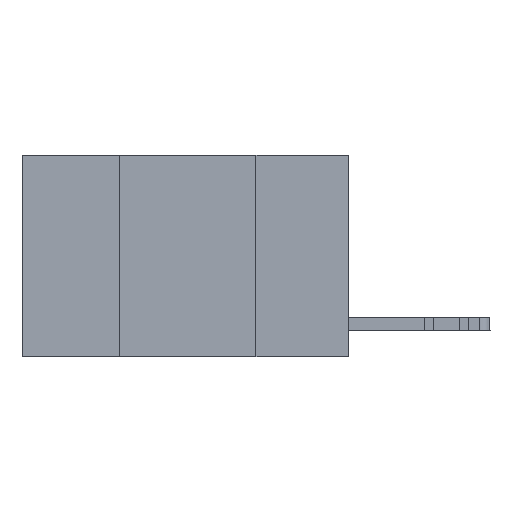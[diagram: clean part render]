
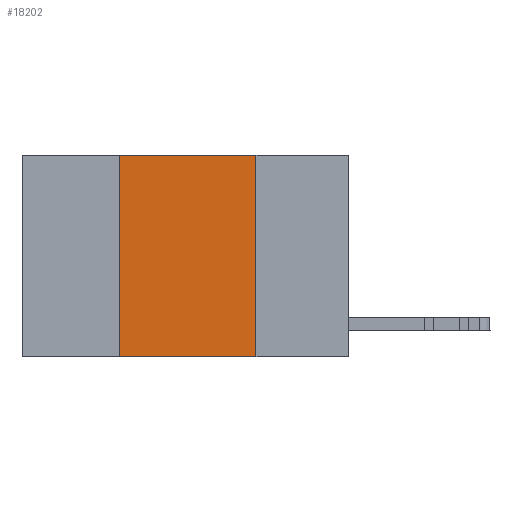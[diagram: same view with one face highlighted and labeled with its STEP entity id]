
A CAD part, left-side view. The second image highlights one B-rep face of the part: STEP entity #18202.
In plain terms, the highlighted planar face has unit normal (-1, 0, 0).
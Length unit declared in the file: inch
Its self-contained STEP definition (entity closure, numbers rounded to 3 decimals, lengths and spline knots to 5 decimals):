
#2142 = LINE ( 'NONE', #16442, #11073 ) ;
#2859 = VERTEX_POINT ( 'NONE', #10514 ) ;
#4257 = ORIENTED_EDGE ( 'NONE', *, *, #20470, .F. ) ;
#4533 = LINE ( 'NONE', #17146, #8910 ) ;
#5981 = PLANE ( 'NONE',  #22032 ) ;
#6725 = LINE ( 'NONE', #23983, #12965 ) ;
#7134 = DIRECTION ( 'NONE',  ( 0., -1., 0. ) ) ;
#8594 = EDGE_LOOP ( 'NONE', ( #9467, #24457, #4257, #24720 ) ) ;
#8910 = VECTOR ( 'NONE', #7134, 39.37008 ) ;
#9030 = CARTESIAN_POINT ( 'NONE',  ( 0., 0.42, -0.37 ) ) ;
#9467 = ORIENTED_EDGE ( 'NONE', *, *, #14985, .F. ) ;
#9581 = LINE ( 'NONE', #13747, #23902 ) ;
#10507 = DIRECTION ( 'NONE',  ( 1., 0., 0. ) ) ;
#10514 = CARTESIAN_POINT ( 'NONE',  ( 0., 0.42, 0. ) ) ;
#11073 = VECTOR ( 'NONE', #25139, 39.37008 ) ;
#11332 = EDGE_CURVE ( 'NONE', #2859, #19741, #4533, .T. ) ;
#12965 = VECTOR ( 'NONE', #14904, 39.37008 ) ;
#13704 = VERTEX_POINT ( 'NONE', #9030 ) ;
#13747 = CARTESIAN_POINT ( 'NONE',  ( 0., 0.6, -0.37 ) ) ;
#14904 = DIRECTION ( 'NONE',  ( 0., 0., -1. ) ) ;
#14985 = EDGE_CURVE ( 'NONE', #19741, #25496, #6725, .T. ) ;
#16442 = CARTESIAN_POINT ( 'NONE',  ( 0., 0.42, 0. ) ) ;
#16849 = CARTESIAN_POINT ( 'NONE',  ( 0., 0.17, -0.37 ) ) ;
#17146 = CARTESIAN_POINT ( 'NONE',  ( 0., 0.6, 0. ) ) ;
#18202 = ADVANCED_FACE ( 'NONE', ( #25062 ), #5981, .F. ) ;
#19572 = CARTESIAN_POINT ( 'NONE',  ( 0., 0.17, 0. ) ) ;
#19741 = VERTEX_POINT ( 'NONE', #19572 ) ;
#20470 = EDGE_CURVE ( 'NONE', #13704, #2859, #2142, .T. ) ;
#20626 = DIRECTION ( 'NONE',  ( 0., -1., 0. ) ) ;
#22032 = AXIS2_PLACEMENT_3D ( 'NONE', #22954, #10507, #23227 ) ;
#22954 = CARTESIAN_POINT ( 'NONE',  ( 0., 0.6, 0. ) ) ;
#23227 = DIRECTION ( 'NONE',  ( 0., 0., -1. ) ) ;
#23902 = VECTOR ( 'NONE', #20626, 39.37008 ) ;
#23983 = CARTESIAN_POINT ( 'NONE',  ( 0., 0.17, 0. ) ) ;
#24457 = ORIENTED_EDGE ( 'NONE', *, *, #11332, .F. ) ;
#24720 = ORIENTED_EDGE ( 'NONE', *, *, #27025, .T. ) ;
#25062 = FACE_OUTER_BOUND ( 'NONE', #8594, .T. ) ;
#25139 = DIRECTION ( 'NONE',  ( 0., 0., 1. ) ) ;
#25496 = VERTEX_POINT ( 'NONE', #16849 ) ;
#27025 = EDGE_CURVE ( 'NONE', #13704, #25496, #9581, .T. ) ;
